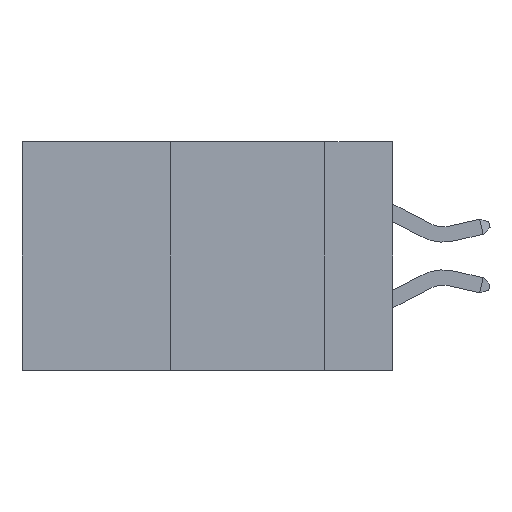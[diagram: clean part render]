
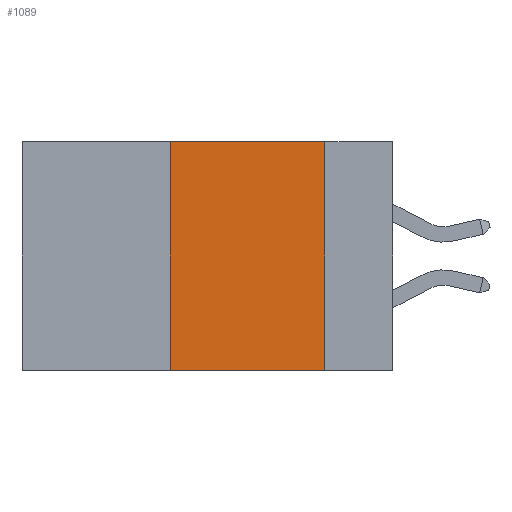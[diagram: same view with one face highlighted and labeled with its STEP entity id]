
A CAD part, left-side view. The second image highlights one B-rep face of the part: STEP entity #1089.
In plain terms, the highlighted planar face has unit normal (-1, 0, 0).
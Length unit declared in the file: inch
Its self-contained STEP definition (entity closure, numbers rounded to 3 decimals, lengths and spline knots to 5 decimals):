
#1089 = ADVANCED_FACE ( 'NONE', ( #14031 ), #20438, .F. ) ;
#1376 = VERTEX_POINT ( 'NONE', #17559 ) ;
#1409 = CARTESIAN_POINT ( 'NONE',  ( 0., 0.36, 0. ) ) ;
#1876 = VERTEX_POINT ( 'NONE', #1409 ) ;
#1984 = LINE ( 'NONE', #6219, #9989 ) ;
#2688 = ORIENTED_EDGE ( 'NONE', *, *, #22653, .T. ) ;
#2928 = AXIS2_PLACEMENT_3D ( 'NONE', #20595, #6452, #16849 ) ;
#3420 = CARTESIAN_POINT ( 'NONE',  ( 0., 0.11, -0.37 ) ) ;
#3928 = EDGE_CURVE ( 'NONE', #5255, #22301, #15849, .T. ) ;
#4325 = DIRECTION ( 'NONE',  ( 0., 0., -1. ) ) ;
#4350 = LINE ( 'NONE', #17669, #18077 ) ;
#4449 = DIRECTION ( 'NONE',  ( 0., -1., 0. ) ) ;
#4493 = DIRECTION ( 'NONE',  ( 0., -1., 0. ) ) ;
#5255 = VERTEX_POINT ( 'NONE', #20365 ) ;
#6219 = CARTESIAN_POINT ( 'NONE',  ( 0., 0.6, 0. ) ) ;
#6452 = DIRECTION ( 'NONE',  ( 1., 0., 0. ) ) ;
#8811 = ORIENTED_EDGE ( 'NONE', *, *, #17515, .F. ) ;
#9989 = VECTOR ( 'NONE', #4449, 39.37008 ) ;
#10217 = VECTOR ( 'NONE', #20335, 39.37008 ) ;
#11360 = CARTESIAN_POINT ( 'NONE',  ( 0., 0.36, 0. ) ) ;
#11811 = EDGE_CURVE ( 'NONE', #1376, #1876, #22573, .T. ) ;
#12394 = ORIENTED_EDGE ( 'NONE', *, *, #11811, .F. ) ;
#14031 = FACE_OUTER_BOUND ( 'NONE', #20946, .T. ) ;
#15240 = ORIENTED_EDGE ( 'NONE', *, *, #3928, .F. ) ;
#15320 = VECTOR ( 'NONE', #4325, 39.37008 ) ;
#15849 = LINE ( 'NONE', #16707, #15320 ) ;
#16707 = CARTESIAN_POINT ( 'NONE',  ( 0., 0.11, 0. ) ) ;
#16849 = DIRECTION ( 'NONE',  ( 0., 0., -1. ) ) ;
#17515 = EDGE_CURVE ( 'NONE', #1876, #5255, #1984, .T. ) ;
#17559 = CARTESIAN_POINT ( 'NONE',  ( 0., 0.36, -0.37 ) ) ;
#17669 = CARTESIAN_POINT ( 'NONE',  ( 0., 0.6, -0.37 ) ) ;
#18077 = VECTOR ( 'NONE', #4493, 39.37008 ) ;
#20335 = DIRECTION ( 'NONE',  ( 0., 0., 1. ) ) ;
#20365 = CARTESIAN_POINT ( 'NONE',  ( 0., 0.11, 0. ) ) ;
#20438 = PLANE ( 'NONE',  #2928 ) ;
#20595 = CARTESIAN_POINT ( 'NONE',  ( 0., 0.6, 0. ) ) ;
#20946 = EDGE_LOOP ( 'NONE', ( #15240, #8811, #12394, #2688 ) ) ;
#22301 = VERTEX_POINT ( 'NONE', #3420 ) ;
#22573 = LINE ( 'NONE', #11360, #10217 ) ;
#22653 = EDGE_CURVE ( 'NONE', #1376, #22301, #4350, .T. ) ;
